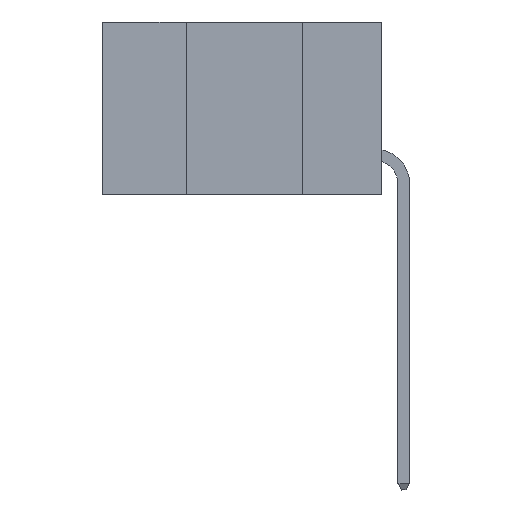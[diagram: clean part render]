
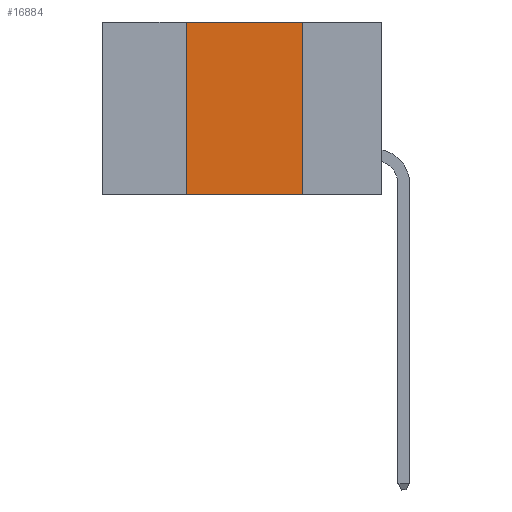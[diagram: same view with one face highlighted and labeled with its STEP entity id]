
A CAD part, left-side view. The second image highlights one B-rep face of the part: STEP entity #16884.
In plain terms, the highlighted planar face has unit normal (-1, 0, 0).
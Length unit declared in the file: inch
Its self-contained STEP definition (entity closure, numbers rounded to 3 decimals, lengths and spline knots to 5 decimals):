
#384 = EDGE_CURVE ( 'NONE', #2926, #24673, #9825, .T. ) ;
#2140 = CARTESIAN_POINT ( 'NONE',  ( 0., 0.42, 0. ) ) ;
#2926 = VERTEX_POINT ( 'NONE', #17432 ) ;
#3704 = CARTESIAN_POINT ( 'NONE',  ( 0., 0.42, -0.37 ) ) ;
#3935 = LINE ( 'NONE', #2140, #10502 ) ;
#5283 = EDGE_CURVE ( 'NONE', #26400, #2926, #22784, .T. ) ;
#5395 = EDGE_CURVE ( 'NONE', #6858, #24673, #12854, .T. ) ;
#6327 = VECTOR ( 'NONE', #11563, 39.37008 ) ;
#6858 = VERTEX_POINT ( 'NONE', #3704 ) ;
#8526 = VECTOR ( 'NONE', #14314, 39.37008 ) ;
#9825 = LINE ( 'NONE', #10104, #8526 ) ;
#10104 = CARTESIAN_POINT ( 'NONE',  ( 0., 0.17, 0. ) ) ;
#10502 = VECTOR ( 'NONE', #19298, 39.37008 ) ;
#11563 = DIRECTION ( 'NONE',  ( 0., -1., 0. ) ) ;
#12854 = LINE ( 'NONE', #16075, #13854 ) ;
#13760 = DIRECTION ( 'NONE',  ( 0., -1., 0. ) ) ;
#13854 = VECTOR ( 'NONE', #13760, 39.37008 ) ;
#14314 = DIRECTION ( 'NONE',  ( 0., 0., -1. ) ) ;
#15116 = ORIENTED_EDGE ( 'NONE', *, *, #24208, .F. ) ;
#16075 = CARTESIAN_POINT ( 'NONE',  ( 0., 0.6, -0.37 ) ) ;
#16533 = PLANE ( 'NONE',  #24387 ) ;
#16884 = ADVANCED_FACE ( 'NONE', ( #27064 ), #16533, .F. ) ;
#17432 = CARTESIAN_POINT ( 'NONE',  ( 0., 0.17, 0. ) ) ;
#18791 = CARTESIAN_POINT ( 'NONE',  ( 0., 0.6, 0. ) ) ;
#19298 = DIRECTION ( 'NONE',  ( 0., 0., 1. ) ) ;
#20374 = CARTESIAN_POINT ( 'NONE',  ( 0., 0.17, -0.37 ) ) ;
#21234 = EDGE_LOOP ( 'NONE', ( #26048, #22909, #15116, #22761 ) ) ;
#22761 = ORIENTED_EDGE ( 'NONE', *, *, #5395, .T. ) ;
#22784 = LINE ( 'NONE', #26088, #6327 ) ;
#22909 = ORIENTED_EDGE ( 'NONE', *, *, #5283, .F. ) ;
#22936 = DIRECTION ( 'NONE',  ( 0., 0., -1. ) ) ;
#23821 = CARTESIAN_POINT ( 'NONE',  ( 0., 0.42, 0. ) ) ;
#24208 = EDGE_CURVE ( 'NONE', #6858, #26400, #3935, .T. ) ;
#24387 = AXIS2_PLACEMENT_3D ( 'NONE', #18791, #27144, #22936 ) ;
#24673 = VERTEX_POINT ( 'NONE', #20374 ) ;
#26048 = ORIENTED_EDGE ( 'NONE', *, *, #384, .F. ) ;
#26088 = CARTESIAN_POINT ( 'NONE',  ( 0., 0.6, 0. ) ) ;
#26400 = VERTEX_POINT ( 'NONE', #23821 ) ;
#27064 = FACE_OUTER_BOUND ( 'NONE', #21234, .T. ) ;
#27144 = DIRECTION ( 'NONE',  ( 1., 0., 0. ) ) ;
